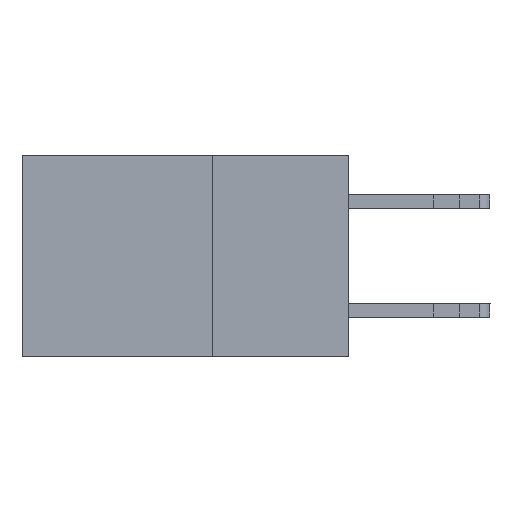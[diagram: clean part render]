
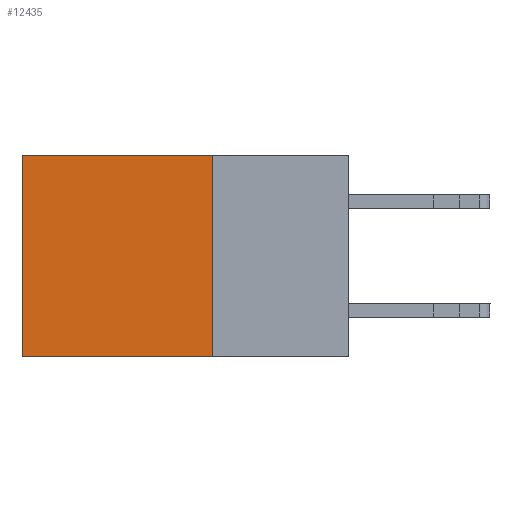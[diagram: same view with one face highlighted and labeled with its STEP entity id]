
A CAD part, left-side view. The second image highlights one B-rep face of the part: STEP entity #12435.
In plain terms, the highlighted planar face has unit normal (-1, 0, 0).
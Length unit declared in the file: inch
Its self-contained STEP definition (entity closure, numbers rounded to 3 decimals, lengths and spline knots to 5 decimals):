
#1079 = VECTOR ( 'NONE', #2869, 39.37008 ) ;
#1119 = DIRECTION ( 'NONE',  ( 0., 1., 0. ) ) ;
#1141 = CARTESIAN_POINT ( 'NONE',  ( 0.298, 0.25, 0. ) ) ;
#1357 = VECTOR ( 'NONE', #1119, 39.37008 ) ;
#1419 = LINE ( 'NONE', #1141, #1079 ) ;
#1535 = CARTESIAN_POINT ( 'NONE',  ( 0.298, 0.25, 0. ) ) ;
#1918 = LINE ( 'NONE', #3833, #4683 ) ;
#2433 = AXIS2_PLACEMENT_3D ( 'NONE', #1535, #8412, #7342 ) ;
#2659 = DIRECTION ( 'NONE',  ( 0., 0., -1. ) ) ;
#2665 = FACE_OUTER_BOUND ( 'NONE', #13472, .T. ) ;
#2869 = DIRECTION ( 'NONE',  ( 0., 0., -1. ) ) ;
#3498 = EDGE_CURVE ( 'NONE', #12797, #3953, #1918, .T. ) ;
#3833 = CARTESIAN_POINT ( 'NONE',  ( 0.298, 0.6, 0. ) ) ;
#3953 = VERTEX_POINT ( 'NONE', #13516 ) ;
#4203 = EDGE_CURVE ( 'NONE', #9975, #3953, #4842, .T. ) ;
#4204 = CARTESIAN_POINT ( 'NONE',  ( 0.298, 0.25, 0. ) ) ;
#4683 = VECTOR ( 'NONE', #2659, 39.37008 ) ;
#4842 = LINE ( 'NONE', #13832, #1357 ) ;
#5172 = ORIENTED_EDGE ( 'NONE', *, *, #14240, .T. ) ;
#5218 = CARTESIAN_POINT ( 'NONE',  ( 0.298, 0.25, 0. ) ) ;
#7342 = DIRECTION ( 'NONE',  ( 0., 0., -1. ) ) ;
#7706 = ORIENTED_EDGE ( 'NONE', *, *, #14162, .F. ) ;
#8398 = LINE ( 'NONE', #5218, #14360 ) ;
#8412 = DIRECTION ( 'NONE',  ( 1., 0., 0. ) ) ;
#8513 = PLANE ( 'NONE',  #2433 ) ;
#8689 = DIRECTION ( 'NONE',  ( 0., 1., 0. ) ) ;
#9109 = ORIENTED_EDGE ( 'NONE', *, *, #3498, .T. ) ;
#9911 = CARTESIAN_POINT ( 'NONE',  ( 0.298, 0.25, -0.37 ) ) ;
#9975 = VERTEX_POINT ( 'NONE', #9911 ) ;
#10778 = ORIENTED_EDGE ( 'NONE', *, *, #4203, .F. ) ;
#11323 = CARTESIAN_POINT ( 'NONE',  ( 0.298, 0.6, 0. ) ) ;
#12435 = ADVANCED_FACE ( 'NONE', ( #2665 ), #8513, .F. ) ;
#12797 = VERTEX_POINT ( 'NONE', #11323 ) ;
#13472 = EDGE_LOOP ( 'NONE', ( #9109, #10778, #7706, #5172 ) ) ;
#13516 = CARTESIAN_POINT ( 'NONE',  ( 0.298, 0.6, -0.37 ) ) ;
#13832 = CARTESIAN_POINT ( 'NONE',  ( 0.298, 0.25, -0.37 ) ) ;
#13841 = VERTEX_POINT ( 'NONE', #4204 ) ;
#14162 = EDGE_CURVE ( 'NONE', #13841, #9975, #1419, .T. ) ;
#14240 = EDGE_CURVE ( 'NONE', #13841, #12797, #8398, .T. ) ;
#14360 = VECTOR ( 'NONE', #8689, 39.37008 ) ;
